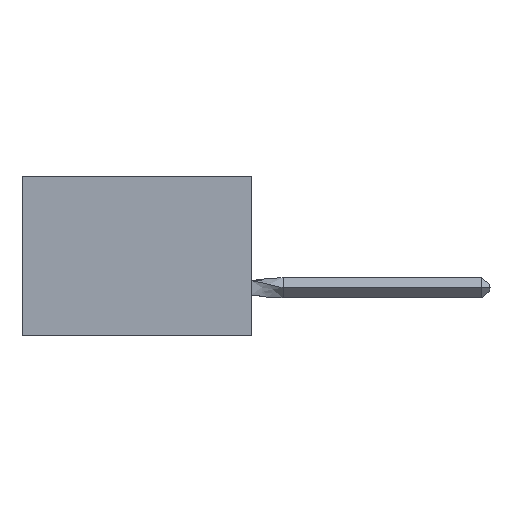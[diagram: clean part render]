
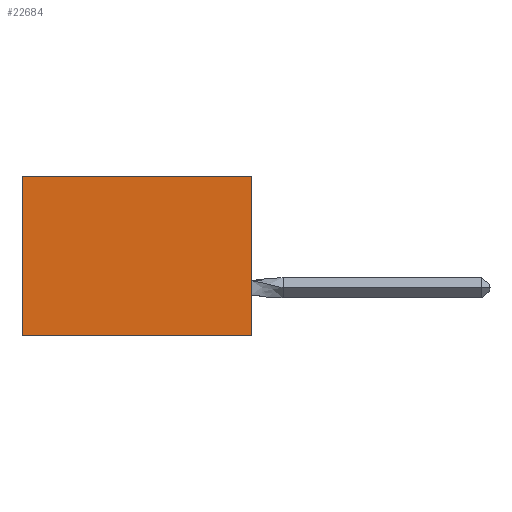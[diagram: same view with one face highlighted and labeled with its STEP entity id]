
A CAD part, left-side view. The second image highlights one B-rep face of the part: STEP entity #22684.
In plain terms, the highlighted planar face has unit normal (-1, 0, 0).
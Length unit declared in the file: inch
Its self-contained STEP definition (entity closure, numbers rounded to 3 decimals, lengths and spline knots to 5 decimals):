
#634 = VECTOR ( 'NONE', #13508, 39.37008 ) ;
#2748 = DIRECTION ( 'NONE',  ( 0., 0., -1. ) ) ;
#2783 = CARTESIAN_POINT ( 'NONE',  ( 0.305, 0.72, -0.5 ) ) ;
#3830 = LINE ( 'NONE', #14086, #5278 ) ;
#3986 = VERTEX_POINT ( 'NONE', #7129 ) ;
#4064 = VERTEX_POINT ( 'NONE', #28045 ) ;
#4718 = ORIENTED_EDGE ( 'NONE', *, *, #14056, .T. ) ;
#4973 = DIRECTION ( 'NONE',  ( 0., 1., 0. ) ) ;
#5278 = VECTOR ( 'NONE', #4973, 39.37008 ) ;
#6244 = ORIENTED_EDGE ( 'NONE', *, *, #16076, .F. ) ;
#6316 = EDGE_CURVE ( 'NONE', #3986, #4064, #15002, .T. ) ;
#7129 = CARTESIAN_POINT ( 'NONE',  ( 0.305, 0., 0. ) ) ;
#7166 = ORIENTED_EDGE ( 'NONE', *, *, #10586, .T. ) ;
#7790 = DIRECTION ( 'NONE',  ( 0., 1., 0. ) ) ;
#8518 = VECTOR ( 'NONE', #2748, 39.37008 ) ;
#8891 = CARTESIAN_POINT ( 'NONE',  ( 0.305, 0.72, -0.5 ) ) ;
#10020 = ORIENTED_EDGE ( 'NONE', *, *, #6316, .F. ) ;
#10586 = EDGE_CURVE ( 'NONE', #3986, #10627, #3830, .T. ) ;
#10627 = VERTEX_POINT ( 'NONE', #16296 ) ;
#13389 = FACE_OUTER_BOUND ( 'NONE', #21231, .T. ) ;
#13470 = DIRECTION ( 'NONE',  ( 1., 0., 0. ) ) ;
#13508 = DIRECTION ( 'NONE',  ( 0., 0., -1. ) ) ;
#13580 = PLANE ( 'NONE',  #28714 ) ;
#14056 = EDGE_CURVE ( 'NONE', #10627, #28234, #20811, .T. ) ;
#14086 = CARTESIAN_POINT ( 'NONE',  ( 0.305, 0., 0. ) ) ;
#15002 = LINE ( 'NONE', #21248, #8518 ) ;
#16076 = EDGE_CURVE ( 'NONE', #4064, #28234, #16305, .T. ) ;
#16296 = CARTESIAN_POINT ( 'NONE',  ( 0.305, 0.72, 0. ) ) ;
#16305 = LINE ( 'NONE', #21586, #17385 ) ;
#17385 = VECTOR ( 'NONE', #7790, 39.37008 ) ;
#18097 = CARTESIAN_POINT ( 'NONE',  ( 0.305, 0., -0.5 ) ) ;
#20811 = LINE ( 'NONE', #8891, #634 ) ;
#21231 = EDGE_LOOP ( 'NONE', ( #4718, #6244, #10020, #7166 ) ) ;
#21248 = CARTESIAN_POINT ( 'NONE',  ( 0.305, 0., -0.5 ) ) ;
#21586 = CARTESIAN_POINT ( 'NONE',  ( 0.305, 0., -0.5 ) ) ;
#22684 = ADVANCED_FACE ( 'NONE', ( #13389 ), #13580, .F. ) ;
#27649 = DIRECTION ( 'NONE',  ( 0., 0., -1. ) ) ;
#28045 = CARTESIAN_POINT ( 'NONE',  ( 0.305, 0., -0.5 ) ) ;
#28234 = VERTEX_POINT ( 'NONE', #2783 ) ;
#28714 = AXIS2_PLACEMENT_3D ( 'NONE', #18097, #13470, #27649 ) ;
